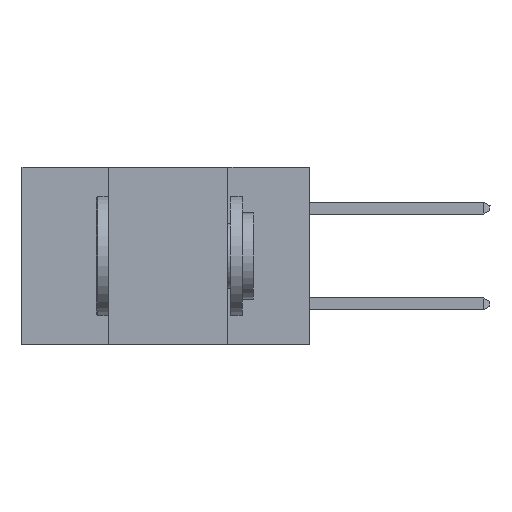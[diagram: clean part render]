
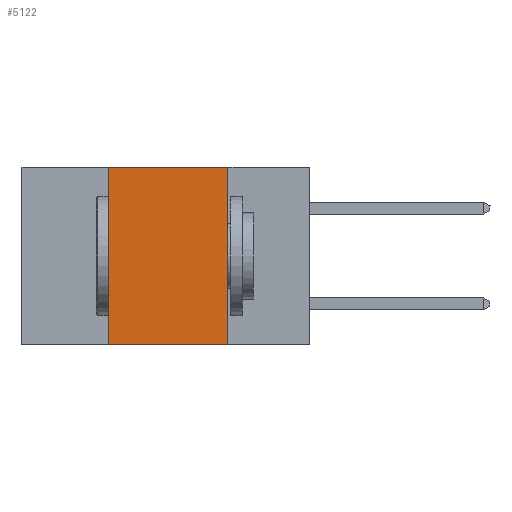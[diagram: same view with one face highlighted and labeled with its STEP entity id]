
A CAD part, left-side view. The second image highlights one B-rep face of the part: STEP entity #5122.
In plain terms, the highlighted planar face has unit normal (-1, 0, 0).
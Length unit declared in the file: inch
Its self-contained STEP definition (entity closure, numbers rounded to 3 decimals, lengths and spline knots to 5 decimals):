
#965 = CARTESIAN_POINT ( 'NONE',  ( 0., 0.42, 0. ) ) ;
#2629 = CARTESIAN_POINT ( 'NONE',  ( 0., 0.17, -0.37 ) ) ;
#4335 = EDGE_CURVE ( 'NONE', #8648, #30815, #33694, .T. ) ;
#5122 = ADVANCED_FACE ( 'NONE', ( #16603 ), #27843, .F. ) ;
#6734 = CARTESIAN_POINT ( 'NONE',  ( 0., 0.6, -0.37 ) ) ;
#6938 = EDGE_CURVE ( 'NONE', #15962, #30815, #18238, .T. ) ;
#8638 = AXIS2_PLACEMENT_3D ( 'NONE', #11344, #23535, #12537 ) ;
#8648 = VERTEX_POINT ( 'NONE', #19419 ) ;
#9004 = DIRECTION ( 'NONE',  ( 0., 0., 1. ) ) ;
#10063 = ORIENTED_EDGE ( 'NONE', *, *, #21091, .F. ) ;
#10650 = VECTOR ( 'NONE', #26304, 39.37008 ) ;
#11344 = CARTESIAN_POINT ( 'NONE',  ( 0., 0.6, 0. ) ) ;
#12421 = DIRECTION ( 'NONE',  ( 0., -1., 0. ) ) ;
#12537 = DIRECTION ( 'NONE',  ( 0., 0., -1. ) ) ;
#12622 = VECTOR ( 'NONE', #9004, 39.37008 ) ;
#12801 = LINE ( 'NONE', #29781, #29841 ) ;
#13279 = ORIENTED_EDGE ( 'NONE', *, *, #22677, .F. ) ;
#15722 = DIRECTION ( 'NONE',  ( 0., -1., 0. ) ) ;
#15856 = CARTESIAN_POINT ( 'NONE',  ( 0., 0.42, 0. ) ) ;
#15962 = VERTEX_POINT ( 'NONE', #36096 ) ;
#16202 = VECTOR ( 'NONE', #12421, 39.37008 ) ;
#16603 = FACE_OUTER_BOUND ( 'NONE', #29826, .T. ) ;
#18238 = LINE ( 'NONE', #32370, #10650 ) ;
#19419 = CARTESIAN_POINT ( 'NONE',  ( 0., 0.42, -0.37 ) ) ;
#21091 = EDGE_CURVE ( 'NONE', #8648, #27555, #26453, .T. ) ;
#22677 = EDGE_CURVE ( 'NONE', #27555, #15962, #12801, .T. ) ;
#23535 = DIRECTION ( 'NONE',  ( 1., 0., 0. ) ) ;
#25853 = ORIENTED_EDGE ( 'NONE', *, *, #4335, .T. ) ;
#26304 = DIRECTION ( 'NONE',  ( 0., 0., -1. ) ) ;
#26453 = LINE ( 'NONE', #965, #12622 ) ;
#27555 = VERTEX_POINT ( 'NONE', #15856 ) ;
#27843 = PLANE ( 'NONE',  #8638 ) ;
#29781 = CARTESIAN_POINT ( 'NONE',  ( 0., 0.6, 0. ) ) ;
#29826 = EDGE_LOOP ( 'NONE', ( #35257, #13279, #10063, #25853 ) ) ;
#29841 = VECTOR ( 'NONE', #15722, 39.37008 ) ;
#30815 = VERTEX_POINT ( 'NONE', #2629 ) ;
#32370 = CARTESIAN_POINT ( 'NONE',  ( 0., 0.17, 0. ) ) ;
#33694 = LINE ( 'NONE', #6734, #16202 ) ;
#35257 = ORIENTED_EDGE ( 'NONE', *, *, #6938, .F. ) ;
#36096 = CARTESIAN_POINT ( 'NONE',  ( 0., 0.17, 0. ) ) ;
